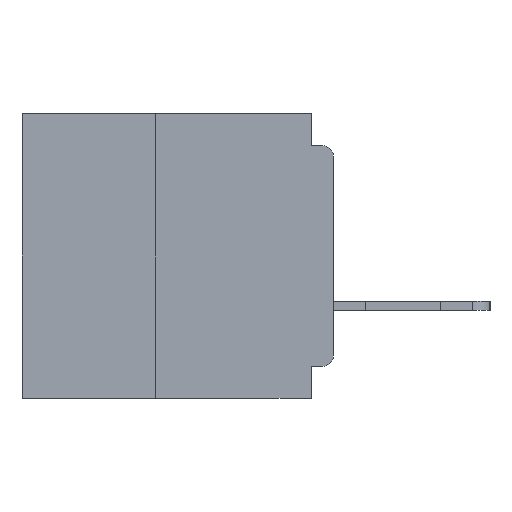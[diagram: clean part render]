
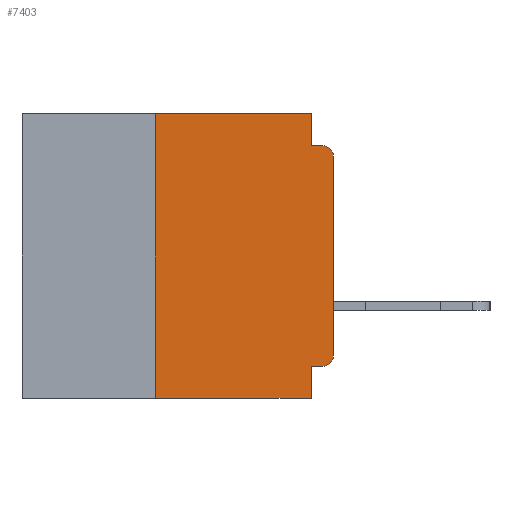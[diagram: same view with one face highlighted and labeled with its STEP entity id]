
A CAD part, left-side view. The second image highlights one B-rep face of the part: STEP entity #7403.
In plain terms, the highlighted planar face has unit normal (-1, 0, 0).
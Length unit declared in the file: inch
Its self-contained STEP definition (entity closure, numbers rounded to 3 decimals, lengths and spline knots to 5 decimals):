
#230 = CARTESIAN_POINT ( 'NONE',  ( 0., 0.437, -0.4 ) ) ;
#306 = CARTESIAN_POINT ( 'NONE',  ( 0., 0., -0.355 ) ) ;
#968 = CARTESIAN_POINT ( 'NONE',  ( 0., 0.015, -0.34 ) ) ;
#2463 = VERTEX_POINT ( 'NONE', #25316 ) ;
#2976 = VECTOR ( 'NONE', #19131, 39.37008 ) ;
#4178 = LINE ( 'NONE', #46415, #2976 ) ;
#4208 = DIRECTION ( 'NONE',  ( 0., -1., 0. ) ) ;
#4814 = VECTOR ( 'NONE', #31369, 39.37008 ) ;
#4946 = DIRECTION ( 'NONE',  ( 0., 0., -1. ) ) ;
#5426 = EDGE_CURVE ( 'NONE', #15901, #14071, #48050, .T. ) ;
#7403 = ADVANCED_FACE ( 'NONE', ( #17304 ), #44574, .F. ) ;
#7665 = CIRCLE ( 'NONE', #8968, 0.015 ) ;
#7898 = CARTESIAN_POINT ( 'NONE',  ( 0., 0., -0.06 ) ) ;
#8866 = VECTOR ( 'NONE', #38033, 39.37008 ) ;
#8968 = AXIS2_PLACEMENT_3D ( 'NONE', #968, #28434, #4946 ) ;
#9614 = DIRECTION ( 'NONE',  ( 0., 0., -1. ) ) ;
#10120 = EDGE_CURVE ( 'NONE', #13512, #15901, #7665, .T. ) ;
#10908 = CARTESIAN_POINT ( 'NONE',  ( 0., 0.031, -0.4 ) ) ;
#13512 = VERTEX_POINT ( 'NONE', #31896 ) ;
#14015 = ORIENTED_EDGE ( 'NONE', *, *, #34793, .F. ) ;
#14064 = CARTESIAN_POINT ( 'NONE',  ( 0., 0.031, -0.045 ) ) ;
#14071 = VERTEX_POINT ( 'NONE', #7898 ) ;
#14587 = CARTESIAN_POINT ( 'NONE',  ( 0., 0.015, -0.06 ) ) ;
#14613 = CARTESIAN_POINT ( 'NONE',  ( 0., 0.437, 0. ) ) ;
#15901 = VERTEX_POINT ( 'NONE', #17982 ) ;
#16404 = VECTOR ( 'NONE', #4208, 39.37008 ) ;
#17105 = ORIENTED_EDGE ( 'NONE', *, *, #28782, .F. ) ;
#17304 = FACE_OUTER_BOUND ( 'NONE', #29032, .T. ) ;
#17601 = LINE ( 'NONE', #10908, #48713 ) ;
#17982 = CARTESIAN_POINT ( 'NONE',  ( 0., 0., -0.34 ) ) ;
#18509 = DIRECTION ( 'NONE',  ( 0., 0., -1. ) ) ;
#19131 = DIRECTION ( 'NONE',  ( 0., 0., 1. ) ) ;
#21284 = DIRECTION ( 'NONE',  ( 0., -1., 0. ) ) ;
#21723 = EDGE_CURVE ( 'NONE', #28592, #2463, #47904, .T. ) ;
#22050 = LINE ( 'NONE', #25218, #30019 ) ;
#25218 = CARTESIAN_POINT ( 'NONE',  ( 0., 0., -0.045 ) ) ;
#25259 = EDGE_CURVE ( 'NONE', #14071, #34682, #45777, .T. ) ;
#25316 = CARTESIAN_POINT ( 'NONE',  ( 0., 0.031, 0. ) ) ;
#25688 = LINE ( 'NONE', #50537, #4814 ) ;
#26642 = DIRECTION ( 'NONE',  ( 0., 0., -1. ) ) ;
#28191 = EDGE_CURVE ( 'NONE', #43311, #28592, #4178, .T. ) ;
#28331 = EDGE_CURVE ( 'NONE', #43311, #43929, #37246, .T. ) ;
#28434 = DIRECTION ( 'NONE',  ( -1., 0., 0. ) ) ;
#28592 = VERTEX_POINT ( 'NONE', #33328 ) ;
#28782 = EDGE_CURVE ( 'NONE', #30589, #43929, #17601, .T. ) ;
#29032 = EDGE_LOOP ( 'NONE', ( #38117, #50665, #47157, #50162, #46586, #33814, #47866, #17105, #14015, #43594 ) ) ;
#29281 = CARTESIAN_POINT ( 'NONE',  ( 0., 0.031, -0.4 ) ) ;
#29793 = VECTOR ( 'NONE', #31540, 39.37008 ) ;
#30019 = VECTOR ( 'NONE', #21284, 39.37008 ) ;
#30589 = VERTEX_POINT ( 'NONE', #31930 ) ;
#31369 = DIRECTION ( 'NONE',  ( 0., 0., -1. ) ) ;
#31540 = DIRECTION ( 'NONE',  ( 0., 1., 0. ) ) ;
#31563 = AXIS2_PLACEMENT_3D ( 'NONE', #14587, #41903, #18509 ) ;
#31896 = CARTESIAN_POINT ( 'NONE',  ( 0., 0.015, -0.355 ) ) ;
#31930 = CARTESIAN_POINT ( 'NONE',  ( 0., 0.031, -0.355 ) ) ;
#32995 = EDGE_CURVE ( 'NONE', #2463, #48859, #25688, .T. ) ;
#33049 = DIRECTION ( 'NONE',  ( 1., 0., 0. ) ) ;
#33204 = CARTESIAN_POINT ( 'NONE',  ( 0., 0., 0. ) ) ;
#33328 = CARTESIAN_POINT ( 'NONE',  ( 0., 0.25, 0. ) ) ;
#33814 = ORIENTED_EDGE ( 'NONE', *, *, #28191, .F. ) ;
#34682 = VERTEX_POINT ( 'NONE', #46494 ) ;
#34793 = EDGE_CURVE ( 'NONE', #13512, #30589, #40107, .T. ) ;
#37246 = LINE ( 'NONE', #230, #16404 ) ;
#37747 = VECTOR ( 'NONE', #41017, 39.37008 ) ;
#38033 = DIRECTION ( 'NONE',  ( 0., -1., 0. ) ) ;
#38117 = ORIENTED_EDGE ( 'NONE', *, *, #5426, .T. ) ;
#40107 = LINE ( 'NONE', #306, #29793 ) ;
#41017 = DIRECTION ( 'NONE',  ( 0., 0., 1. ) ) ;
#41903 = DIRECTION ( 'NONE',  ( -1., 0., 0. ) ) ;
#43311 = VERTEX_POINT ( 'NONE', #46057 ) ;
#43594 = ORIENTED_EDGE ( 'NONE', *, *, #10120, .T. ) ;
#43929 = VERTEX_POINT ( 'NONE', #29281 ) ;
#44574 = PLANE ( 'NONE',  #47423 ) ;
#45777 = CIRCLE ( 'NONE', #31563, 0.015 ) ;
#46057 = CARTESIAN_POINT ( 'NONE',  ( 0., 0.25, -0.4 ) ) ;
#46415 = CARTESIAN_POINT ( 'NONE',  ( 0., 0.25, -0.4 ) ) ;
#46494 = CARTESIAN_POINT ( 'NONE',  ( 0., 0.015, -0.045 ) ) ;
#46586 = ORIENTED_EDGE ( 'NONE', *, *, #21723, .F. ) ;
#47157 = ORIENTED_EDGE ( 'NONE', *, *, #48766, .F. ) ;
#47423 = AXIS2_PLACEMENT_3D ( 'NONE', #48472, #33049, #9614 ) ;
#47866 = ORIENTED_EDGE ( 'NONE', *, *, #28331, .T. ) ;
#47904 = LINE ( 'NONE', #14613, #8866 ) ;
#48050 = LINE ( 'NONE', #33204, #37747 ) ;
#48472 = CARTESIAN_POINT ( 'NONE',  ( 0., 0.437, 0. ) ) ;
#48713 = VECTOR ( 'NONE', #26642, 39.37008 ) ;
#48766 = EDGE_CURVE ( 'NONE', #48859, #34682, #22050, .T. ) ;
#48859 = VERTEX_POINT ( 'NONE', #14064 ) ;
#50162 = ORIENTED_EDGE ( 'NONE', *, *, #32995, .F. ) ;
#50537 = CARTESIAN_POINT ( 'NONE',  ( 0., 0.031, 0. ) ) ;
#50665 = ORIENTED_EDGE ( 'NONE', *, *, #25259, .T. ) ;
